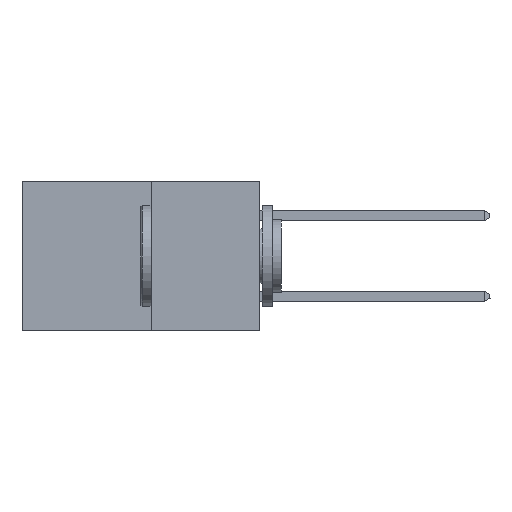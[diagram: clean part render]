
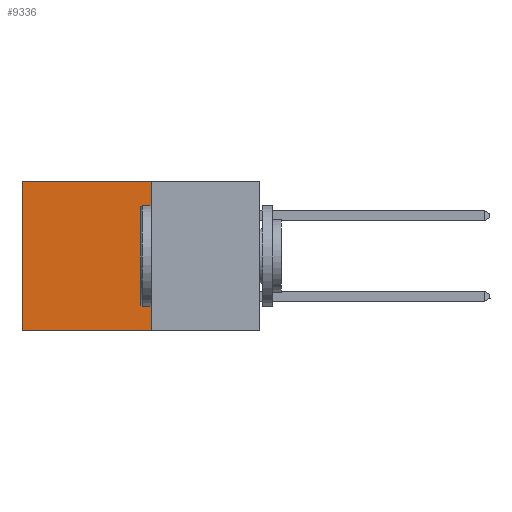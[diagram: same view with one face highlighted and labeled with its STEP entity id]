
A CAD part, left-side view. The second image highlights one B-rep face of the part: STEP entity #9336.
In plain terms, the highlighted planar face has unit normal (-1, 0, 0).
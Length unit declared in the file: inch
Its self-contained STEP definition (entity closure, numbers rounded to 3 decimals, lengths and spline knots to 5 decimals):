
#40 = ORIENTED_EDGE ( 'NONE', *, *, #16291, .T. ) ;
#385 = CARTESIAN_POINT ( 'NONE',  ( 0.277, 0.27, 0. ) ) ;
#2418 = DIRECTION ( 'NONE',  ( 0., 1., 0. ) ) ;
#3262 = LINE ( 'NONE', #385, #18818 ) ;
#3307 = AXIS2_PLACEMENT_3D ( 'NONE', #16853, #18870, #6772 ) ;
#4552 = ORIENTED_EDGE ( 'NONE', *, *, #6811, .F. ) ;
#4608 = ORIENTED_EDGE ( 'NONE', *, *, #8537, .T. ) ;
#6772 = DIRECTION ( 'NONE',  ( 0., 0., -1. ) ) ;
#6811 = EDGE_CURVE ( 'NONE', #14891, #9313, #7220, .T. ) ;
#7220 = LINE ( 'NONE', #19887, #7873 ) ;
#7873 = VECTOR ( 'NONE', #20177, 39.37008 ) ;
#8537 = EDGE_CURVE ( 'NONE', #25912, #9313, #9010, .T. ) ;
#8696 = EDGE_CURVE ( 'NONE', #19730, #14891, #10578, .T. ) ;
#9010 = LINE ( 'NONE', #21571, #19124 ) ;
#9313 = VERTEX_POINT ( 'NONE', #16685 ) ;
#9336 = ADVANCED_FACE ( 'NONE', ( #11492 ), #14846, .F. ) ;
#10578 = LINE ( 'NONE', #17473, #25902 ) ;
#11492 = FACE_OUTER_BOUND ( 'NONE', #22830, .T. ) ;
#14846 = PLANE ( 'NONE',  #3307 ) ;
#14891 = VERTEX_POINT ( 'NONE', #22407 ) ;
#16291 = EDGE_CURVE ( 'NONE', #19730, #25912, #3262, .T. ) ;
#16685 = CARTESIAN_POINT ( 'NONE',  ( 0.277, 0.59, -0.37 ) ) ;
#16853 = CARTESIAN_POINT ( 'NONE',  ( 0.277, 0.27, -0.37 ) ) ;
#17325 = DIRECTION ( 'NONE',  ( 0., 0., -1. ) ) ;
#17473 = CARTESIAN_POINT ( 'NONE',  ( 0.277, 0.27, -0.37 ) ) ;
#18818 = VECTOR ( 'NONE', #2418, 39.37008 ) ;
#18870 = DIRECTION ( 'NONE',  ( 1., 0., 0. ) ) ;
#19124 = VECTOR ( 'NONE', #21344, 39.37008 ) ;
#19210 = CARTESIAN_POINT ( 'NONE',  ( 0.277, 0.59, 0. ) ) ;
#19730 = VERTEX_POINT ( 'NONE', #25621 ) ;
#19887 = CARTESIAN_POINT ( 'NONE',  ( 0.277, 0.27, -0.37 ) ) ;
#20177 = DIRECTION ( 'NONE',  ( 0., 1., 0. ) ) ;
#21344 = DIRECTION ( 'NONE',  ( 0., 0., -1. ) ) ;
#21571 = CARTESIAN_POINT ( 'NONE',  ( 0.277, 0.59, -0.37 ) ) ;
#21996 = ORIENTED_EDGE ( 'NONE', *, *, #8696, .F. ) ;
#22407 = CARTESIAN_POINT ( 'NONE',  ( 0.277, 0.27, -0.37 ) ) ;
#22830 = EDGE_LOOP ( 'NONE', ( #4608, #4552, #21996, #40 ) ) ;
#25621 = CARTESIAN_POINT ( 'NONE',  ( 0.277, 0.27, 0. ) ) ;
#25902 = VECTOR ( 'NONE', #17325, 39.37008 ) ;
#25912 = VERTEX_POINT ( 'NONE', #19210 ) ;
